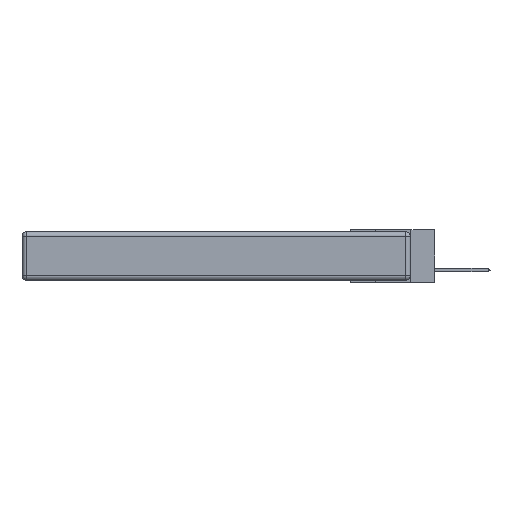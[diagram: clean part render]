
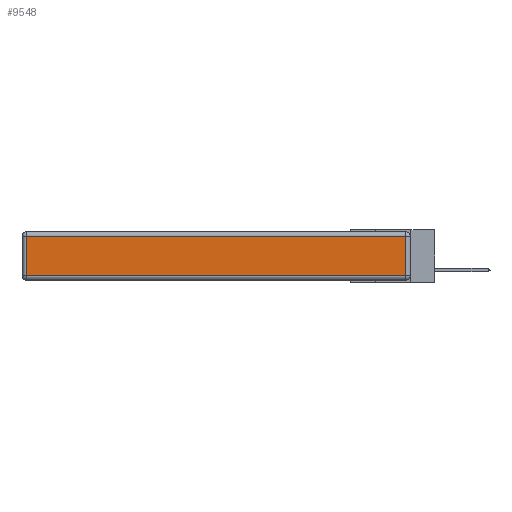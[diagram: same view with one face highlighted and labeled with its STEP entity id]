
A CAD part, left-side view. The second image highlights one B-rep face of the part: STEP entity #9548.
In plain terms, the highlighted planar face has unit normal (-1, 0, 0).
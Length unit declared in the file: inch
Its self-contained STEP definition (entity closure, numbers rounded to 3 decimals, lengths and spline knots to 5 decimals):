
#1720 = FACE_OUTER_BOUND ( 'NONE', #15955, .T. ) ;
#1998 = VECTOR ( 'NONE', #14709, 39.37008 ) ;
#2911 = DIRECTION ( 'NONE',  ( 0., 1., 0. ) ) ;
#5794 = CARTESIAN_POINT ( 'NONE',  ( 0., 0.03, -0.313 ) ) ;
#6009 = PLANE ( 'NONE',  #23305 ) ;
#7187 = ORIENTED_EDGE ( 'NONE', *, *, #20330, .T. ) ;
#7305 = LINE ( 'NONE', #19319, #17912 ) ;
#7358 = VECTOR ( 'NONE', #22507, 39.37008 ) ;
#8681 = EDGE_CURVE ( 'NONE', #20405, #15224, #14851, .T. ) ;
#9012 = VERTEX_POINT ( 'NONE', #15139 ) ;
#9548 = ADVANCED_FACE ( 'NONE', ( #1720 ), #6009, .T. ) ;
#10215 = CARTESIAN_POINT ( 'NONE',  ( 0., 2.72, -0.03 ) ) ;
#10359 = DIRECTION ( 'NONE',  ( -1., 0., 0. ) ) ;
#11211 = EDGE_CURVE ( 'NONE', #26474, #20405, #7305, .T. ) ;
#12598 = DIRECTION ( 'NONE',  ( 0., 0., 1. ) ) ;
#12624 = DIRECTION ( 'NONE',  ( 0., 0., 1. ) ) ;
#12920 = EDGE_CURVE ( 'NONE', #15224, #9012, #23522, .T. ) ;
#14709 = DIRECTION ( 'NONE',  ( 0., 0., -1. ) ) ;
#14851 = LINE ( 'NONE', #18828, #25065 ) ;
#15139 = CARTESIAN_POINT ( 'NONE',  ( 0., 2.72, -0.313 ) ) ;
#15224 = VERTEX_POINT ( 'NONE', #10215 ) ;
#15319 = CARTESIAN_POINT ( 'NONE',  ( 0., 0.03, -0.03 ) ) ;
#15955 = EDGE_LOOP ( 'NONE', ( #7187, #19076, #26720, #22514 ) ) ;
#17912 = VECTOR ( 'NONE', #12598, 39.37008 ) ;
#18828 = CARTESIAN_POINT ( 'NONE',  ( 0., 2.75, -0.03 ) ) ;
#19076 = ORIENTED_EDGE ( 'NONE', *, *, #11211, .T. ) ;
#19319 = CARTESIAN_POINT ( 'NONE',  ( 0., 0.03, -0.343 ) ) ;
#20330 = EDGE_CURVE ( 'NONE', #9012, #26474, #20785, .T. ) ;
#20405 = VERTEX_POINT ( 'NONE', #15319 ) ;
#20785 = LINE ( 'NONE', #26616, #7358 ) ;
#21610 = CARTESIAN_POINT ( 'NONE',  ( 0., 2.72, -0.343 ) ) ;
#21614 = CARTESIAN_POINT ( 'NONE',  ( 0., 0., -0.343 ) ) ;
#22507 = DIRECTION ( 'NONE',  ( 0., -1., 0. ) ) ;
#22514 = ORIENTED_EDGE ( 'NONE', *, *, #12920, .T. ) ;
#23305 = AXIS2_PLACEMENT_3D ( 'NONE', #21614, #10359, #12624 ) ;
#23522 = LINE ( 'NONE', #21610, #1998 ) ;
#25065 = VECTOR ( 'NONE', #2911, 39.37008 ) ;
#26474 = VERTEX_POINT ( 'NONE', #5794 ) ;
#26616 = CARTESIAN_POINT ( 'NONE',  ( 0., 0., -0.313 ) ) ;
#26720 = ORIENTED_EDGE ( 'NONE', *, *, #8681, .T. ) ;
